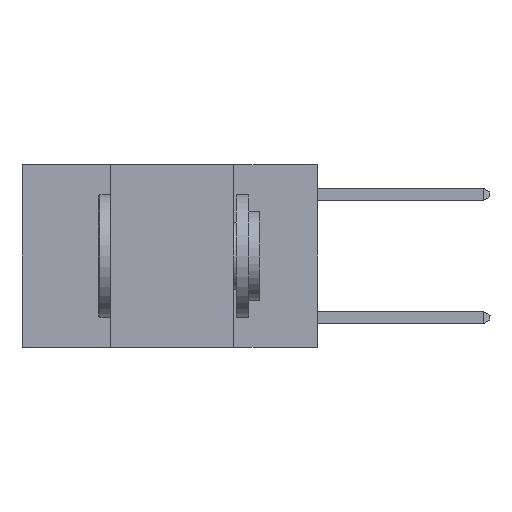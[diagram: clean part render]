
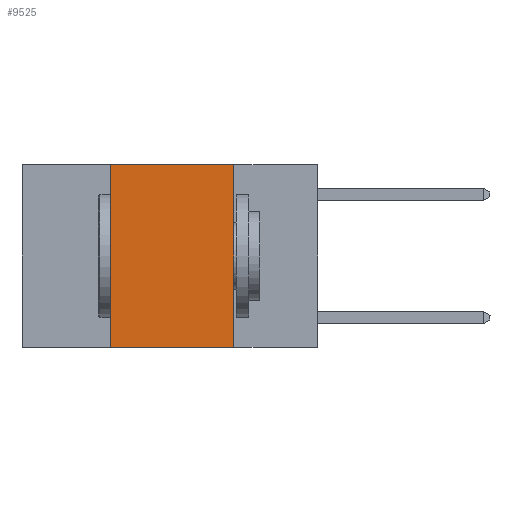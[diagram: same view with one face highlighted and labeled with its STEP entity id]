
A CAD part, left-side view. The second image highlights one B-rep face of the part: STEP entity #9525.
In plain terms, the highlighted planar face has unit normal (-1, 0, 0).
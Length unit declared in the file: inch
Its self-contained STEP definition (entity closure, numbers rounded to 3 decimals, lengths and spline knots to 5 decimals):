
#274 = AXIS2_PLACEMENT_3D ( 'NONE', #15284, #7526, #16562 ) ;
#484 = CARTESIAN_POINT ( 'NONE',  ( 0., 0.17, -0.37 ) ) ;
#1179 = CARTESIAN_POINT ( 'NONE',  ( 0., 0.42, -0.37 ) ) ;
#1533 = LINE ( 'NONE', #1876, #11526 ) ;
#1876 = CARTESIAN_POINT ( 'NONE',  ( 0., 0.42, 0. ) ) ;
#1894 = CARTESIAN_POINT ( 'NONE',  ( 0., 0.6, 0. ) ) ;
#2283 = PLANE ( 'NONE',  #274 ) ;
#2475 = EDGE_CURVE ( 'NONE', #11611, #3991, #15182, .T. ) ;
#2969 = VECTOR ( 'NONE', #12298, 39.37008 ) ;
#3017 = CARTESIAN_POINT ( 'NONE',  ( 0., 0.17, 0. ) ) ;
#3225 = VECTOR ( 'NONE', #10829, 39.37008 ) ;
#3233 = CARTESIAN_POINT ( 'NONE',  ( 0., 0.17, 0. ) ) ;
#3311 = EDGE_CURVE ( 'NONE', #12395, #7947, #9886, .T. ) ;
#3991 = VERTEX_POINT ( 'NONE', #484 ) ;
#4584 = DIRECTION ( 'NONE',  ( 0., 0., 1. ) ) ;
#5481 = FACE_OUTER_BOUND ( 'NONE', #9950, .T. ) ;
#6675 = LINE ( 'NONE', #3017, #3225 ) ;
#7526 = DIRECTION ( 'NONE',  ( 1., 0., 0. ) ) ;
#7892 = VECTOR ( 'NONE', #10492, 39.37008 ) ;
#7947 = VERTEX_POINT ( 'NONE', #3233 ) ;
#8316 = ORIENTED_EDGE ( 'NONE', *, *, #14997, .F. ) ;
#8712 = ORIENTED_EDGE ( 'NONE', *, *, #3311, .F. ) ;
#9525 = ADVANCED_FACE ( 'NONE', ( #5481 ), #2283, .F. ) ;
#9886 = LINE ( 'NONE', #1894, #2969 ) ;
#9950 = EDGE_LOOP ( 'NONE', ( #8316, #8712, #12164, #12557 ) ) ;
#10218 = CARTESIAN_POINT ( 'NONE',  ( 0., 0.6, -0.37 ) ) ;
#10492 = DIRECTION ( 'NONE',  ( 0., -1., 0. ) ) ;
#10829 = DIRECTION ( 'NONE',  ( 0., 0., -1. ) ) ;
#11526 = VECTOR ( 'NONE', #4584, 39.37008 ) ;
#11611 = VERTEX_POINT ( 'NONE', #1179 ) ;
#12164 = ORIENTED_EDGE ( 'NONE', *, *, #16030, .F. ) ;
#12298 = DIRECTION ( 'NONE',  ( 0., -1., 0. ) ) ;
#12395 = VERTEX_POINT ( 'NONE', #13450 ) ;
#12557 = ORIENTED_EDGE ( 'NONE', *, *, #2475, .T. ) ;
#13450 = CARTESIAN_POINT ( 'NONE',  ( 0., 0.42, 0. ) ) ;
#14997 = EDGE_CURVE ( 'NONE', #7947, #3991, #6675, .T. ) ;
#15182 = LINE ( 'NONE', #10218, #7892 ) ;
#15284 = CARTESIAN_POINT ( 'NONE',  ( 0., 0.6, 0. ) ) ;
#16030 = EDGE_CURVE ( 'NONE', #11611, #12395, #1533, .T. ) ;
#16562 = DIRECTION ( 'NONE',  ( 0., 0., -1. ) ) ;
